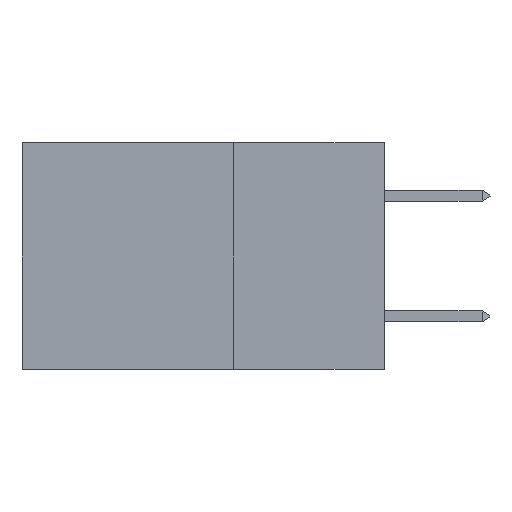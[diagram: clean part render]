
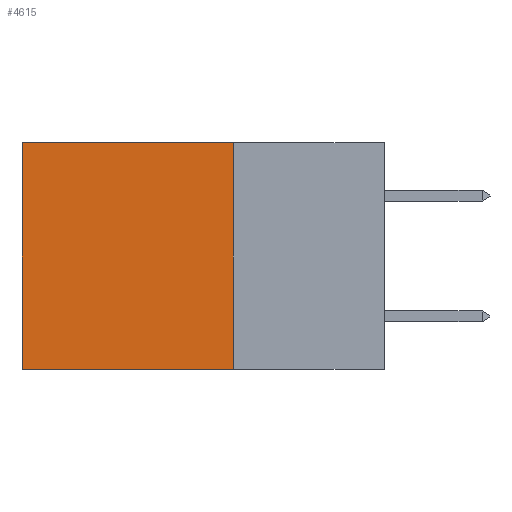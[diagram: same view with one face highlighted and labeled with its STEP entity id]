
A CAD part, left-side view. The second image highlights one B-rep face of the part: STEP entity #4615.
In plain terms, the highlighted planar face has unit normal (-1, 0, 0).
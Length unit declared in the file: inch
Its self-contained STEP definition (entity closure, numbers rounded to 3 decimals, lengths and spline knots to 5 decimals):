
#18 = CARTESIAN_POINT ( 'NONE',  ( 0.2875, 0.25, -0.375 ) ) ;
#1043 = VECTOR ( 'NONE', #6743, 39.37008 ) ;
#1715 = VECTOR ( 'NONE', #5830, 39.37008 ) ;
#1750 = AXIS2_PLACEMENT_3D ( 'NONE', #9957, #13303, #2758 ) ;
#1832 = ORIENTED_EDGE ( 'NONE', *, *, #6619, .T. ) ;
#1959 = VECTOR ( 'NONE', #2787, 39.37008 ) ;
#1992 = ORIENTED_EDGE ( 'NONE', *, *, #9109, .T. ) ;
#2073 = EDGE_LOOP ( 'NONE', ( #1992, #4925, #13284, #1832 ) ) ;
#2758 = DIRECTION ( 'NONE',  ( 0., 0., -1. ) ) ;
#2787 = DIRECTION ( 'NONE',  ( 0., 1., 0. ) ) ;
#4234 = CARTESIAN_POINT ( 'NONE',  ( 0.2875, 0.6, 0. ) ) ;
#4615 = ADVANCED_FACE ( 'NONE', ( #8922 ), #5968, .F. ) ;
#4925 = ORIENTED_EDGE ( 'NONE', *, *, #7681, .F. ) ;
#5615 = VERTEX_POINT ( 'NONE', #18 ) ;
#5766 = LINE ( 'NONE', #9828, #1043 ) ;
#5830 = DIRECTION ( 'NONE',  ( 0., 0., -1. ) ) ;
#5968 = PLANE ( 'NONE',  #1750 ) ;
#6213 = CARTESIAN_POINT ( 'NONE',  ( 0.2875, 0.6, -0.375 ) ) ;
#6418 = CARTESIAN_POINT ( 'NONE',  ( 0.2875, 0.25, -0.375 ) ) ;
#6619 = EDGE_CURVE ( 'NONE', #9104, #9323, #5766, .T. ) ;
#6714 = EDGE_CURVE ( 'NONE', #9104, #5615, #7452, .T. ) ;
#6743 = DIRECTION ( 'NONE',  ( 0., 1., 0. ) ) ;
#7452 = LINE ( 'NONE', #6418, #1715 ) ;
#7681 = EDGE_CURVE ( 'NONE', #5615, #8715, #12098, .T. ) ;
#8519 = DIRECTION ( 'NONE',  ( 0., 0., -1. ) ) ;
#8715 = VERTEX_POINT ( 'NONE', #12666 ) ;
#8922 = FACE_OUTER_BOUND ( 'NONE', #2073, .T. ) ;
#9104 = VERTEX_POINT ( 'NONE', #10337 ) ;
#9109 = EDGE_CURVE ( 'NONE', #9323, #8715, #12574, .T. ) ;
#9323 = VERTEX_POINT ( 'NONE', #4234 ) ;
#9828 = CARTESIAN_POINT ( 'NONE',  ( 0.2875, 0.25, 0. ) ) ;
#9957 = CARTESIAN_POINT ( 'NONE',  ( 0.2875, 0.25, -0.375 ) ) ;
#10337 = CARTESIAN_POINT ( 'NONE',  ( 0.2875, 0.25, 0. ) ) ;
#10865 = VECTOR ( 'NONE', #8519, 39.37008 ) ;
#12098 = LINE ( 'NONE', #13401, #1959 ) ;
#12574 = LINE ( 'NONE', #6213, #10865 ) ;
#12666 = CARTESIAN_POINT ( 'NONE',  ( 0.2875, 0.6, -0.375 ) ) ;
#13284 = ORIENTED_EDGE ( 'NONE', *, *, #6714, .F. ) ;
#13303 = DIRECTION ( 'NONE',  ( 1., 0., 0. ) ) ;
#13401 = CARTESIAN_POINT ( 'NONE',  ( 0.2875, 0.25, -0.375 ) ) ;
